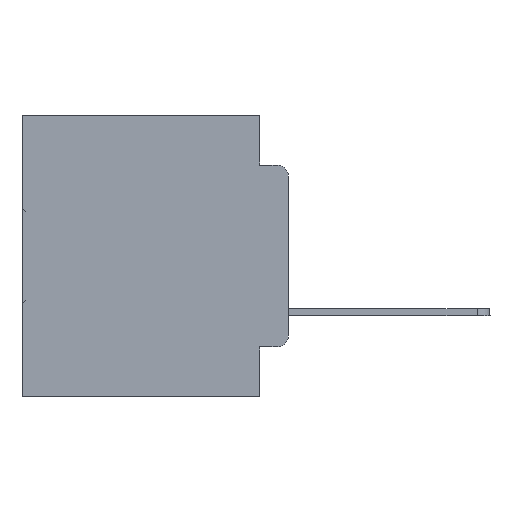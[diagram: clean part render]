
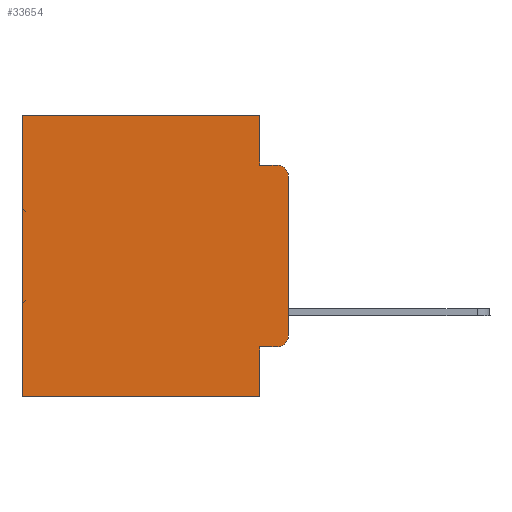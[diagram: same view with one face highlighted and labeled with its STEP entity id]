
A CAD part, left-side view. The second image highlights one B-rep face of the part: STEP entity #33654.
In plain terms, the highlighted planar face has unit normal (-1, 0, 0).
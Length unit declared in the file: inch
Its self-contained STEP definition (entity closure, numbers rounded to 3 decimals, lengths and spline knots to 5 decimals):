
#378 = DIRECTION ( 'NONE',  ( 0., 1., 0. ) ) ;
#512 = ORIENTED_EDGE ( 'NONE', *, *, #18642, .F. ) ;
#976 = VECTOR ( 'NONE', #18367, 39.37008 ) ;
#1336 = AXIS2_PLACEMENT_3D ( 'NONE', #26798, #13506, #2475 ) ;
#1659 = ORIENTED_EDGE ( 'NONE', *, *, #28478, .T. ) ;
#1987 = VECTOR ( 'NONE', #9867, 39.37008 ) ;
#2333 = EDGE_CURVE ( 'NONE', #24196, #23413, #23379, .T. ) ;
#2425 = EDGE_LOOP ( 'NONE', ( #23736, #26230, #21442, #24400, #8704, #20926, #27277, #512, #24671, #1659 ) ) ;
#2475 = DIRECTION ( 'NONE',  ( 0., 0., -1. ) ) ;
#3934 = CARTESIAN_POINT ( 'NONE',  ( 0.298, 0., 0. ) ) ;
#4529 = EDGE_CURVE ( 'NONE', #29723, #23413, #22389, .T. ) ;
#4745 = DIRECTION ( 'NONE',  ( 0., -1., 0. ) ) ;
#4840 = EDGE_CURVE ( 'NONE', #31255, #17830, #30265, .T. ) ;
#5412 = CARTESIAN_POINT ( 'NONE',  ( 0.298, 0., -0.5 ) ) ;
#6059 = DIRECTION ( 'NONE',  ( 0., 0., -1. ) ) ;
#6726 = LINE ( 'NONE', #25168, #31170 ) ;
#7018 = DIRECTION ( 'NONE',  ( 0., 0., -1. ) ) ;
#7279 = VECTOR ( 'NONE', #7018, 39.37008 ) ;
#7291 = LINE ( 'NONE', #23014, #1987 ) ;
#7495 = CARTESIAN_POINT ( 'NONE',  ( 0.298, 0.051, 0. ) ) ;
#7894 = EDGE_CURVE ( 'NONE', #23091, #31629, #6726, .T. ) ;
#8704 = ORIENTED_EDGE ( 'NONE', *, *, #24813, .T. ) ;
#8796 = LINE ( 'NONE', #7495, #976 ) ;
#9044 = CARTESIAN_POINT ( 'NONE',  ( 0.298, 0.051, 0. ) ) ;
#9785 = LINE ( 'NONE', #3934, #7279 ) ;
#9867 = DIRECTION ( 'NONE',  ( 0., 1., 0. ) ) ;
#9968 = CARTESIAN_POINT ( 'NONE',  ( 0.298, 0.051, -0.4115 ) ) ;
#10477 = CARTESIAN_POINT ( 'NONE',  ( 0.298, 0.051, -0.5 ) ) ;
#10816 = VECTOR ( 'NONE', #17390, 39.37008 ) ;
#11587 = DIRECTION ( 'NONE',  ( 0., 0., -1. ) ) ;
#12000 = DIRECTION ( 'NONE',  ( 0., -1., 0. ) ) ;
#12088 = CARTESIAN_POINT ( 'NONE',  ( 0.298, 0.051, -0.0885 ) ) ;
#13105 = VECTOR ( 'NONE', #24877, 39.37008 ) ;
#13288 = VECTOR ( 'NONE', #4745, 39.37008 ) ;
#13506 = DIRECTION ( 'NONE',  ( -1., 0., 0. ) ) ;
#14250 = PLANE ( 'NONE',  #16431 ) ;
#15602 = LINE ( 'NONE', #9044, #13105 ) ;
#16431 = AXIS2_PLACEMENT_3D ( 'NONE', #30327, #27396, #11587 ) ;
#16589 = CIRCLE ( 'NONE', #18751, 0.02 ) ;
#17280 = CARTESIAN_POINT ( 'NONE',  ( 0.298, 0.473, 0. ) ) ;
#17390 = DIRECTION ( 'NONE',  ( 0., 0., -1. ) ) ;
#17830 = VERTEX_POINT ( 'NONE', #29701 ) ;
#18367 = DIRECTION ( 'NONE',  ( 0., 0., -1. ) ) ;
#18642 = EDGE_CURVE ( 'NONE', #31255, #24196, #15602, .T. ) ;
#18688 = FACE_OUTER_BOUND ( 'NONE', #2425, .T. ) ;
#18751 = AXIS2_PLACEMENT_3D ( 'NONE', #24298, #27090, #6059 ) ;
#20926 = ORIENTED_EDGE ( 'NONE', *, *, #4529, .T. ) ;
#21143 = EDGE_CURVE ( 'NONE', #31219, #31629, #30351, .T. ) ;
#21216 = CARTESIAN_POINT ( 'NONE',  ( 0.298, 0.473, 0. ) ) ;
#21442 = ORIENTED_EDGE ( 'NONE', *, *, #7894, .F. ) ;
#22389 = LINE ( 'NONE', #17280, #10816 ) ;
#22551 = VECTOR ( 'NONE', #378, 39.37008 ) ;
#23014 = CARTESIAN_POINT ( 'NONE',  ( 0.298, 0., 0. ) ) ;
#23091 = VERTEX_POINT ( 'NONE', #12088 ) ;
#23379 = LINE ( 'NONE', #5412, #22551 ) ;
#23413 = VERTEX_POINT ( 'NONE', #32751 ) ;
#23736 = ORIENTED_EDGE ( 'NONE', *, *, #31381, .F. ) ;
#24196 = VERTEX_POINT ( 'NONE', #10477 ) ;
#24240 = VERTEX_POINT ( 'NONE', #33921 ) ;
#24298 = CARTESIAN_POINT ( 'NONE',  ( 0.298, 0.02, -0.3915 ) ) ;
#24400 = ORIENTED_EDGE ( 'NONE', *, *, #27861, .F. ) ;
#24671 = ORIENTED_EDGE ( 'NONE', *, *, #4840, .T. ) ;
#24813 = EDGE_CURVE ( 'NONE', #24240, #29723, #7291, .T. ) ;
#24877 = DIRECTION ( 'NONE',  ( 0., 0., -1. ) ) ;
#25168 = CARTESIAN_POINT ( 'NONE',  ( 0.298, 0.051, -0.0885 ) ) ;
#26230 = ORIENTED_EDGE ( 'NONE', *, *, #21143, .T. ) ;
#26798 = CARTESIAN_POINT ( 'NONE',  ( 0.298, 0.02, -0.1085 ) ) ;
#27090 = DIRECTION ( 'NONE',  ( -1., 0., 0. ) ) ;
#27277 = ORIENTED_EDGE ( 'NONE', *, *, #2333, .F. ) ;
#27396 = DIRECTION ( 'NONE',  ( 1., 0., 0. ) ) ;
#27861 = EDGE_CURVE ( 'NONE', #24240, #23091, #8796, .T. ) ;
#28453 = CARTESIAN_POINT ( 'NONE',  ( 0.298, 0.051, -0.4115 ) ) ;
#28478 = EDGE_CURVE ( 'NONE', #17830, #29178, #16589, .T. ) ;
#29178 = VERTEX_POINT ( 'NONE', #32033 ) ;
#29372 = CARTESIAN_POINT ( 'NONE',  ( 0.298, 0.02, -0.0885 ) ) ;
#29701 = CARTESIAN_POINT ( 'NONE',  ( 0.298, 0.02, -0.4115 ) ) ;
#29723 = VERTEX_POINT ( 'NONE', #21216 ) ;
#30265 = LINE ( 'NONE', #28453, #13288 ) ;
#30327 = CARTESIAN_POINT ( 'NONE',  ( 0.298, 0., 0. ) ) ;
#30351 = CIRCLE ( 'NONE', #1336, 0.02 ) ;
#31170 = VECTOR ( 'NONE', #12000, 39.37008 ) ;
#31219 = VERTEX_POINT ( 'NONE', #33248 ) ;
#31255 = VERTEX_POINT ( 'NONE', #9968 ) ;
#31381 = EDGE_CURVE ( 'NONE', #31219, #29178, #9785, .T. ) ;
#31629 = VERTEX_POINT ( 'NONE', #29372 ) ;
#32033 = CARTESIAN_POINT ( 'NONE',  ( 0.298, 0., -0.3915 ) ) ;
#32751 = CARTESIAN_POINT ( 'NONE',  ( 0.298, 0.473, -0.5 ) ) ;
#33248 = CARTESIAN_POINT ( 'NONE',  ( 0.298, 0., -0.1085 ) ) ;
#33654 = ADVANCED_FACE ( 'NONE', ( #18688 ), #14250, .F. ) ;
#33921 = CARTESIAN_POINT ( 'NONE',  ( 0.298, 0.051, 0. ) ) ;
